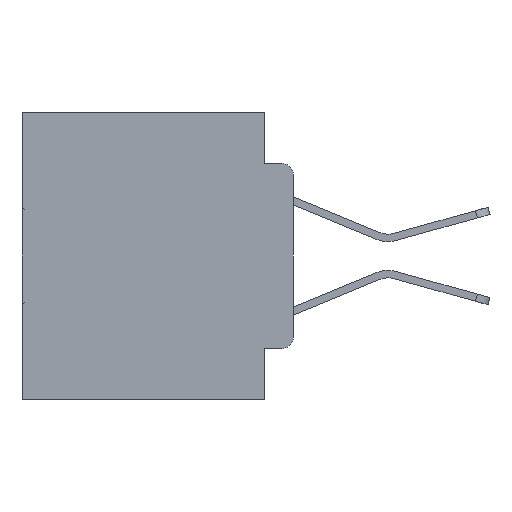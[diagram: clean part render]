
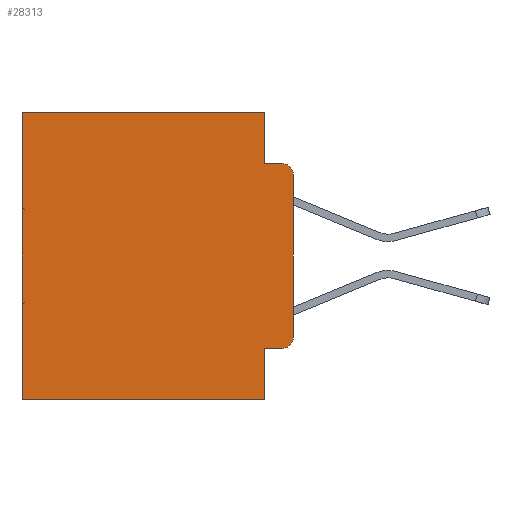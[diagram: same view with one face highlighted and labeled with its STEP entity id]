
A CAD part, left-side view. The second image highlights one B-rep face of the part: STEP entity #28313.
In plain terms, the highlighted planar face has unit normal (-1, 0, 0).
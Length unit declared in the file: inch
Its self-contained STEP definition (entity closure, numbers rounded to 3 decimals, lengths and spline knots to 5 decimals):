
#503 = CARTESIAN_POINT ( 'NONE',  ( 0.298, 0., 0. ) ) ;
#1782 = EDGE_CURVE ( 'NONE', #8299, #1892, #11194, .T. ) ;
#1892 = VERTEX_POINT ( 'NONE', #16745 ) ;
#2103 = EDGE_CURVE ( 'NONE', #8414, #4021, #25560, .T. ) ;
#2141 = CIRCLE ( 'NONE', #23087, 0.02 ) ;
#2318 = ORIENTED_EDGE ( 'NONE', *, *, #19171, .F. ) ;
#2575 = CARTESIAN_POINT ( 'NONE',  ( 0.298, 0.02, -0.3915 ) ) ;
#3184 = DIRECTION ( 'NONE',  ( 0., 0., -1. ) ) ;
#3389 = CARTESIAN_POINT ( 'NONE',  ( 0.298, 0.473, 0. ) ) ;
#3675 = EDGE_CURVE ( 'NONE', #7590, #10649, #27413, .T. ) ;
#3679 = CARTESIAN_POINT ( 'NONE',  ( 0.298, 0., -0.1085 ) ) ;
#3920 = EDGE_CURVE ( 'NONE', #11330, #10649, #32754, .T. ) ;
#4021 = VERTEX_POINT ( 'NONE', #21833 ) ;
#5236 = VECTOR ( 'NONE', #12825, 39.37008 ) ;
#5248 = DIRECTION ( 'NONE',  ( 0., 0., -1. ) ) ;
#5785 = ORIENTED_EDGE ( 'NONE', *, *, #20965, .T. ) ;
#6800 = ORIENTED_EDGE ( 'NONE', *, *, #2103, .F. ) ;
#7350 = CIRCLE ( 'NONE', #20621, 0.02 ) ;
#7590 = VERTEX_POINT ( 'NONE', #15945 ) ;
#7985 = LINE ( 'NONE', #22716, #20731 ) ;
#8299 = VERTEX_POINT ( 'NONE', #21183 ) ;
#8414 = VERTEX_POINT ( 'NONE', #3679 ) ;
#9974 = VECTOR ( 'NONE', #18052, 39.37008 ) ;
#10174 = VERTEX_POINT ( 'NONE', #14072 ) ;
#10249 = EDGE_CURVE ( 'NONE', #8414, #14806, #7350, .T. ) ;
#10527 = CARTESIAN_POINT ( 'NONE',  ( 0.298, 0.051, 0. ) ) ;
#10649 = VERTEX_POINT ( 'NONE', #26577 ) ;
#10920 = FACE_OUTER_BOUND ( 'NONE', #28243, .T. ) ;
#11194 = LINE ( 'NONE', #20059, #17957 ) ;
#11330 = VERTEX_POINT ( 'NONE', #31374 ) ;
#11530 = ORIENTED_EDGE ( 'NONE', *, *, #25299, .T. ) ;
#11793 = LINE ( 'NONE', #32452, #19331 ) ;
#12250 = CARTESIAN_POINT ( 'NONE',  ( 0.298, 0.02, -0.0885 ) ) ;
#12680 = CARTESIAN_POINT ( 'NONE',  ( 0.298, 0.02, -0.4115 ) ) ;
#12825 = DIRECTION ( 'NONE',  ( 0., 0., -1. ) ) ;
#13766 = ORIENTED_EDGE ( 'NONE', *, *, #19802, .T. ) ;
#14072 = CARTESIAN_POINT ( 'NONE',  ( 0.298, 0.051, -0.4115 ) ) ;
#14129 = VECTOR ( 'NONE', #28147, 39.37008 ) ;
#14393 = CARTESIAN_POINT ( 'NONE',  ( 0.298, 0.02, -0.1085 ) ) ;
#14806 = VERTEX_POINT ( 'NONE', #12250 ) ;
#15012 = DIRECTION ( 'NONE',  ( 0., 1., 0. ) ) ;
#15945 = CARTESIAN_POINT ( 'NONE',  ( 0.298, 0.473, 0. ) ) ;
#16011 = VECTOR ( 'NONE', #26610, 39.37008 ) ;
#16089 = PLANE ( 'NONE',  #30222 ) ;
#16163 = CARTESIAN_POINT ( 'NONE',  ( 0.298, 0., -0.5 ) ) ;
#16745 = CARTESIAN_POINT ( 'NONE',  ( 0.298, 0.051, -0.0885 ) ) ;
#16927 = DIRECTION ( 'NONE',  ( 0., 0., -1. ) ) ;
#17957 = VECTOR ( 'NONE', #20026, 39.37008 ) ;
#18052 = DIRECTION ( 'NONE',  ( 0., -1., 0. ) ) ;
#18621 = DIRECTION ( 'NONE',  ( 1., 0., 0. ) ) ;
#18670 = ORIENTED_EDGE ( 'NONE', *, *, #10249, .T. ) ;
#19171 = EDGE_CURVE ( 'NONE', #1892, #14806, #7985, .T. ) ;
#19331 = VECTOR ( 'NONE', #15012, 39.37008 ) ;
#19802 = EDGE_CURVE ( 'NONE', #10174, #32366, #29281, .T. ) ;
#20026 = DIRECTION ( 'NONE',  ( 0., 0., -1. ) ) ;
#20044 = LINE ( 'NONE', #10527, #14129 ) ;
#20059 = CARTESIAN_POINT ( 'NONE',  ( 0.298, 0.051, 0. ) ) ;
#20580 = DIRECTION ( 'NONE',  ( -1., 0., 0. ) ) ;
#20621 = AXIS2_PLACEMENT_3D ( 'NONE', #14393, #31856, #16927 ) ;
#20731 = VECTOR ( 'NONE', #25229, 39.37008 ) ;
#20743 = VECTOR ( 'NONE', #27840, 39.37008 ) ;
#20870 = ORIENTED_EDGE ( 'NONE', *, *, #28199, .F. ) ;
#20965 = EDGE_CURVE ( 'NONE', #8299, #7590, #11793, .T. ) ;
#21183 = CARTESIAN_POINT ( 'NONE',  ( 0.298, 0.051, 0. ) ) ;
#21632 = ORIENTED_EDGE ( 'NONE', *, *, #3920, .F. ) ;
#21833 = CARTESIAN_POINT ( 'NONE',  ( 0.298, 0., -0.3915 ) ) ;
#22538 = ORIENTED_EDGE ( 'NONE', *, *, #3675, .T. ) ;
#22716 = CARTESIAN_POINT ( 'NONE',  ( 0.298, 0.051, -0.0885 ) ) ;
#23087 = AXIS2_PLACEMENT_3D ( 'NONE', #2575, #20580, #5248 ) ;
#25229 = DIRECTION ( 'NONE',  ( 0., -1., 0. ) ) ;
#25299 = EDGE_CURVE ( 'NONE', #32366, #4021, #2141, .T. ) ;
#25440 = ORIENTED_EDGE ( 'NONE', *, *, #1782, .F. ) ;
#25560 = LINE ( 'NONE', #32058, #5236 ) ;
#26577 = CARTESIAN_POINT ( 'NONE',  ( 0.298, 0.473, -0.5 ) ) ;
#26610 = DIRECTION ( 'NONE',  ( 0., 1., 0. ) ) ;
#27413 = LINE ( 'NONE', #3389, #20743 ) ;
#27840 = DIRECTION ( 'NONE',  ( 0., 0., -1. ) ) ;
#28147 = DIRECTION ( 'NONE',  ( 0., 0., -1. ) ) ;
#28199 = EDGE_CURVE ( 'NONE', #10174, #11330, #20044, .T. ) ;
#28243 = EDGE_LOOP ( 'NONE', ( #6800, #18670, #2318, #25440, #5785, #22538, #21632, #20870, #13766, #11530 ) ) ;
#28313 = ADVANCED_FACE ( 'NONE', ( #10920 ), #16089, .F. ) ;
#29281 = LINE ( 'NONE', #32935, #9974 ) ;
#30222 = AXIS2_PLACEMENT_3D ( 'NONE', #503, #18621, #3184 ) ;
#31374 = CARTESIAN_POINT ( 'NONE',  ( 0.298, 0.051, -0.5 ) ) ;
#31856 = DIRECTION ( 'NONE',  ( -1., 0., 0. ) ) ;
#32058 = CARTESIAN_POINT ( 'NONE',  ( 0.298, 0., 0. ) ) ;
#32366 = VERTEX_POINT ( 'NONE', #12680 ) ;
#32452 = CARTESIAN_POINT ( 'NONE',  ( 0.298, 0., 0. ) ) ;
#32754 = LINE ( 'NONE', #16163, #16011 ) ;
#32935 = CARTESIAN_POINT ( 'NONE',  ( 0.298, 0.051, -0.4115 ) ) ;
